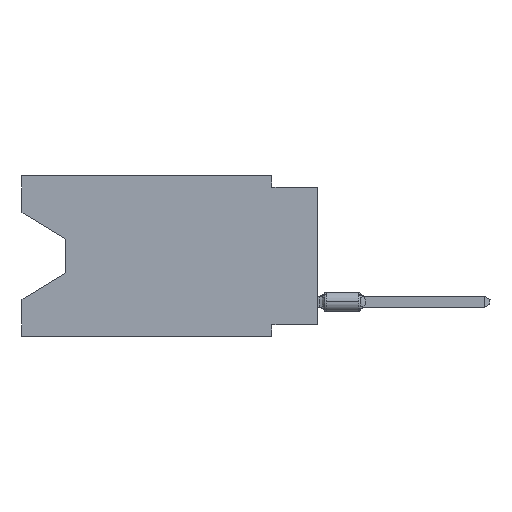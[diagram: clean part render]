
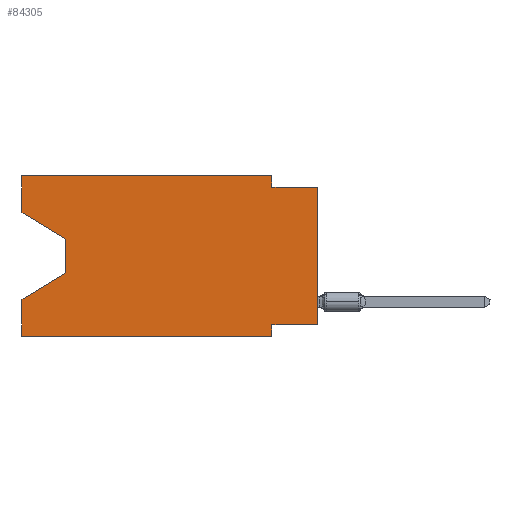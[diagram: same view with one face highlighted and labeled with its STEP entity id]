
A CAD part, left-side view. The second image highlights one B-rep face of the part: STEP entity #84305.
In plain terms, the highlighted planar face has unit normal (-1, 0, 0).
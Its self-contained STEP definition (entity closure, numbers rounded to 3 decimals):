
#361 = DIRECTION ( 'NONE',  ( 0., -1., 0. ) ) ;
#727 = VECTOR ( 'NONE', #361, 1000. ) ;
#1566 = VERTEX_POINT ( 'NONE', #15031 ) ;
#4179 = ORIENTED_EDGE ( 'NONE', *, *, #20501, .T. ) ;
#5708 = LINE ( 'NONE', #83109, #75441 ) ;
#6481 = CARTESIAN_POINT ( 'NONE',  ( 0., 0., -8.255 ) ) ;
#6913 = CARTESIAN_POINT ( 'NONE',  ( 0., 2.54, 0. ) ) ;
#7247 = LINE ( 'NONE', #84204, #10791 ) ;
#7674 = CARTESIAN_POINT ( 'NONE',  ( 0., 16.383, 0. ) ) ;
#8246 = CARTESIAN_POINT ( 'NONE',  ( 0., 13.97, -3.505 ) ) ;
#9141 = CARTESIAN_POINT ( 'NONE',  ( 0., 0., -0.635 ) ) ;
#9406 = CARTESIAN_POINT ( 'NONE',  ( 0., 16.383, 0. ) ) ;
#10642 = EDGE_CURVE ( 'NONE', #17881, #74499, #87040, .T. ) ;
#10791 = VECTOR ( 'NONE', #13678, 1000. ) ;
#11034 = VERTEX_POINT ( 'NONE', #24644 ) ;
#11353 = VERTEX_POINT ( 'NONE', #64367 ) ;
#12327 = DIRECTION ( 'NONE',  ( 0., 0., -1. ) ) ;
#13678 = DIRECTION ( 'NONE',  ( 0., -1., 0. ) ) ;
#15031 = CARTESIAN_POINT ( 'NONE',  ( 0., 13.97, -5.385 ) ) ;
#16472 = AXIS2_PLACEMENT_3D ( 'NONE', #62957, #71176, #77589 ) ;
#16919 = DIRECTION ( 'NONE',  ( 0., 0., 1. ) ) ;
#16925 = VECTOR ( 'NONE', #16919, 1000. ) ;
#17881 = VERTEX_POINT ( 'NONE', #6481 ) ;
#19026 = ORIENTED_EDGE ( 'NONE', *, *, #45461, .T. ) ;
#19173 = LINE ( 'NONE', #32468, #64835 ) ;
#20090 = ORIENTED_EDGE ( 'NONE', *, *, #45445, .F. ) ;
#20401 = ORIENTED_EDGE ( 'NONE', *, *, #58693, .F. ) ;
#20501 = EDGE_CURVE ( 'NONE', #11353, #69612, #32467, .T. ) ;
#22227 = CARTESIAN_POINT ( 'NONE',  ( 0., 16.383, -8.89 ) ) ;
#24644 = CARTESIAN_POINT ( 'NONE',  ( 0., 16.383, 0. ) ) ;
#24777 = ORIENTED_EDGE ( 'NONE', *, *, #77662, .F. ) ;
#25166 = DIRECTION ( 'NONE',  ( 0., -1., 0. ) ) ;
#25720 = VECTOR ( 'NONE', #70003, 1000. ) ;
#27279 = ORIENTED_EDGE ( 'NONE', *, *, #32190, .T. ) ;
#27637 = EDGE_CURVE ( 'NONE', #11353, #11034, #44656, .T. ) ;
#29047 = PLANE ( 'NONE',  #16472 ) ;
#32190 = EDGE_CURVE ( 'NONE', #69612, #1566, #78758, .T. ) ;
#32467 = LINE ( 'NONE', #81495, #49777 ) ;
#32468 = CARTESIAN_POINT ( 'NONE',  ( 0., 2.54, -8.89 ) ) ;
#33746 = CARTESIAN_POINT ( 'NONE',  ( 0., 0., -0.635 ) ) ;
#33893 = EDGE_LOOP ( 'NONE', ( #4179, #27279, #44045, #20401, #19026, #20090, #50137, #90305, #24777, #37149, #61155, #89162 ) ) ;
#34283 = VERTEX_POINT ( 'NONE', #89159 ) ;
#35885 = CARTESIAN_POINT ( 'NONE',  ( 0., 0., 0. ) ) ;
#37076 = LINE ( 'NONE', #79672, #16925 ) ;
#37149 = ORIENTED_EDGE ( 'NONE', *, *, #88966, .F. ) ;
#37305 = VERTEX_POINT ( 'NONE', #6913 ) ;
#37805 = VERTEX_POINT ( 'NONE', #22227 ) ;
#40281 = VECTOR ( 'NONE', #59708, 1000. ) ;
#40482 = VECTOR ( 'NONE', #84735, 1000. ) ;
#42056 = LINE ( 'NONE', #42954, #25720 ) ;
#42438 = VERTEX_POINT ( 'NONE', #46876 ) ;
#42513 = DIRECTION ( 'NONE',  ( 0., 0., 1. ) ) ;
#42954 = CARTESIAN_POINT ( 'NONE',  ( 0., 0., -8.255 ) ) ;
#44045 = ORIENTED_EDGE ( 'NONE', *, *, #47661, .T. ) ;
#44656 = LINE ( 'NONE', #9406, #73050 ) ;
#45445 = EDGE_CURVE ( 'NONE', #34283, #89026, #19173, .T. ) ;
#45461 = EDGE_CURVE ( 'NONE', #37805, #89026, #7247, .T. ) ;
#46876 = CARTESIAN_POINT ( 'NONE',  ( 0., 2.54, -0.635 ) ) ;
#47661 = EDGE_CURVE ( 'NONE', #1566, #89124, #5708, .T. ) ;
#48253 = DIRECTION ( 'NONE',  ( 0., 0.855, -0.519 ) ) ;
#49777 = VECTOR ( 'NONE', #54908, 1000. ) ;
#49782 = LINE ( 'NONE', #7674, #727 ) ;
#50137 = ORIENTED_EDGE ( 'NONE', *, *, #75487, .F. ) ;
#50558 = FACE_OUTER_BOUND ( 'NONE', #33893, .T. ) ;
#50812 = CARTESIAN_POINT ( 'NONE',  ( 0., 13.97, -3.505 ) ) ;
#54908 = DIRECTION ( 'NONE',  ( 0., -0.855, -0.519 ) ) ;
#56800 = VECTOR ( 'NONE', #56946, 1000. ) ;
#56946 = DIRECTION ( 'NONE',  ( 0., 0., 1. ) ) ;
#57865 = EDGE_CURVE ( 'NONE', #11034, #37305, #49782, .T. ) ;
#58693 = EDGE_CURVE ( 'NONE', #37805, #89124, #37076, .T. ) ;
#59708 = DIRECTION ( 'NONE',  ( 0., 0., -1. ) ) ;
#61155 = ORIENTED_EDGE ( 'NONE', *, *, #57865, .F. ) ;
#62863 = CARTESIAN_POINT ( 'NONE',  ( 0., 16.383, -6.852 ) ) ;
#62957 = CARTESIAN_POINT ( 'NONE',  ( 0., 16.383, 0. ) ) ;
#64367 = CARTESIAN_POINT ( 'NONE',  ( 0., 16.383, -2.038 ) ) ;
#64835 = VECTOR ( 'NONE', #12327, 1000. ) ;
#66192 = VECTOR ( 'NONE', #25166, 1000. ) ;
#67472 = CARTESIAN_POINT ( 'NONE',  ( 0., 2.54, -8.89 ) ) ;
#69612 = VERTEX_POINT ( 'NONE', #50812 ) ;
#70003 = DIRECTION ( 'NONE',  ( 0., 1., 0. ) ) ;
#71176 = DIRECTION ( 'NONE',  ( 1., 0., 0. ) ) ;
#73050 = VECTOR ( 'NONE', #42513, 1000. ) ;
#74499 = VERTEX_POINT ( 'NONE', #33746 ) ;
#74794 = LINE ( 'NONE', #80326, #40281 ) ;
#75441 = VECTOR ( 'NONE', #48253, 1000. ) ;
#75487 = EDGE_CURVE ( 'NONE', #17881, #34283, #42056, .T. ) ;
#77589 = DIRECTION ( 'NONE',  ( 0., 0., -1. ) ) ;
#77662 = EDGE_CURVE ( 'NONE', #42438, #74499, #80576, .T. ) ;
#78758 = LINE ( 'NONE', #8246, #40482 ) ;
#79672 = CARTESIAN_POINT ( 'NONE',  ( 0., 16.383, 0. ) ) ;
#80326 = CARTESIAN_POINT ( 'NONE',  ( 0., 2.54, 0. ) ) ;
#80576 = LINE ( 'NONE', #9141, #66192 ) ;
#81495 = CARTESIAN_POINT ( 'NONE',  ( 0., 16.383, -2.038 ) ) ;
#83109 = CARTESIAN_POINT ( 'NONE',  ( 0., 13.97, -5.385 ) ) ;
#84204 = CARTESIAN_POINT ( 'NONE',  ( 0., 16.383, -8.89 ) ) ;
#84305 = ADVANCED_FACE ( 'NONE', ( #50558 ), #29047, .F. ) ;
#84735 = DIRECTION ( 'NONE',  ( 0., 0., -1. ) ) ;
#87040 = LINE ( 'NONE', #35885, #56800 ) ;
#88966 = EDGE_CURVE ( 'NONE', #37305, #42438, #74794, .T. ) ;
#89026 = VERTEX_POINT ( 'NONE', #67472 ) ;
#89124 = VERTEX_POINT ( 'NONE', #62863 ) ;
#89159 = CARTESIAN_POINT ( 'NONE',  ( 0., 2.54, -8.255 ) ) ;
#89162 = ORIENTED_EDGE ( 'NONE', *, *, #27637, .F. ) ;
#90305 = ORIENTED_EDGE ( 'NONE', *, *, #10642, .T. ) ;
